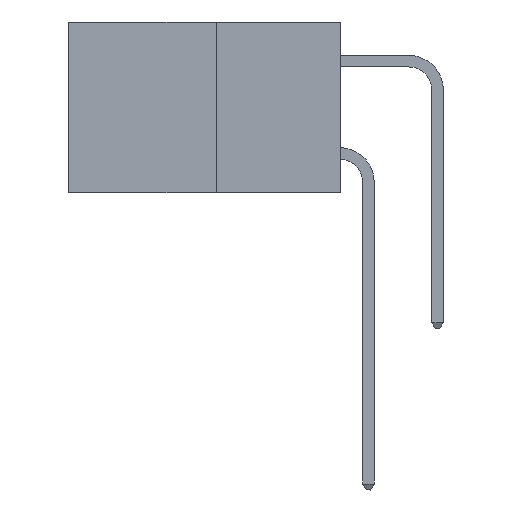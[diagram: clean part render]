
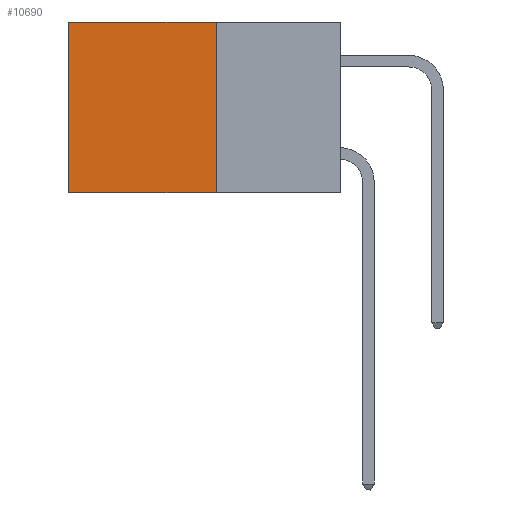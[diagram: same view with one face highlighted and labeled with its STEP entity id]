
A CAD part, left-side view. The second image highlights one B-rep face of the part: STEP entity #10690.
In plain terms, the highlighted planar face has unit normal (-1, 0, 0).
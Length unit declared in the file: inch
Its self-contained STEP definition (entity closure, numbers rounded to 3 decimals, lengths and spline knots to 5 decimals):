
#396 = VECTOR ( 'NONE', #9815, 39.37008 ) ;
#742 = LINE ( 'NONE', #11860, #396 ) ;
#830 = CARTESIAN_POINT ( 'NONE',  ( 0.277, 0.27, 0. ) ) ;
#871 = VECTOR ( 'NONE', #12965, 39.37008 ) ;
#910 = LINE ( 'NONE', #12043, #7142 ) ;
#1106 = CARTESIAN_POINT ( 'NONE',  ( 0.277, 0.59, -0.37 ) ) ;
#1610 = CARTESIAN_POINT ( 'NONE',  ( 0.277, 0.27, -0.37 ) ) ;
#1911 = CARTESIAN_POINT ( 'NONE',  ( 0.277, 0.27, -0.37 ) ) ;
#3246 = DIRECTION ( 'NONE',  ( 1., 0., 0. ) ) ;
#3521 = ORIENTED_EDGE ( 'NONE', *, *, #8546, .T. ) ;
#6115 = VERTEX_POINT ( 'NONE', #1106 ) ;
#6602 = VECTOR ( 'NONE', #10240, 39.37008 ) ;
#6980 = AXIS2_PLACEMENT_3D ( 'NONE', #10043, #3246, #11067 ) ;
#7105 = LINE ( 'NONE', #1911, #871 ) ;
#7142 = VECTOR ( 'NONE', #12002, 39.37008 ) ;
#7728 = EDGE_CURVE ( 'NONE', #10656, #13367, #910, .T. ) ;
#7829 = ORIENTED_EDGE ( 'NONE', *, *, #13526, .F. ) ;
#7856 = PLANE ( 'NONE',  #6980 ) ;
#7890 = CARTESIAN_POINT ( 'NONE',  ( 0.277, 0.59, 0. ) ) ;
#7922 = ORIENTED_EDGE ( 'NONE', *, *, #7728, .F. ) ;
#7990 = CARTESIAN_POINT ( 'NONE',  ( 0.277, 0.59, -0.37 ) ) ;
#8546 = EDGE_CURVE ( 'NONE', #14292, #6115, #9184, .T. ) ;
#9184 = LINE ( 'NONE', #7990, #6602 ) ;
#9752 = ORIENTED_EDGE ( 'NONE', *, *, #11866, .T. ) ;
#9815 = DIRECTION ( 'NONE',  ( 0., 1., 0. ) ) ;
#10043 = CARTESIAN_POINT ( 'NONE',  ( 0.277, 0.27, -0.37 ) ) ;
#10128 = EDGE_LOOP ( 'NONE', ( #3521, #7829, #7922, #9752 ) ) ;
#10240 = DIRECTION ( 'NONE',  ( 0., 0., -1. ) ) ;
#10656 = VERTEX_POINT ( 'NONE', #830 ) ;
#10690 = ADVANCED_FACE ( 'NONE', ( #13609 ), #7856, .F. ) ;
#11067 = DIRECTION ( 'NONE',  ( 0., 0., -1. ) ) ;
#11860 = CARTESIAN_POINT ( 'NONE',  ( 0.277, 0.27, 0. ) ) ;
#11866 = EDGE_CURVE ( 'NONE', #10656, #14292, #742, .T. ) ;
#12002 = DIRECTION ( 'NONE',  ( 0., 0., -1. ) ) ;
#12043 = CARTESIAN_POINT ( 'NONE',  ( 0.277, 0.27, -0.37 ) ) ;
#12965 = DIRECTION ( 'NONE',  ( 0., 1., 0. ) ) ;
#13367 = VERTEX_POINT ( 'NONE', #1610 ) ;
#13526 = EDGE_CURVE ( 'NONE', #13367, #6115, #7105, .T. ) ;
#13609 = FACE_OUTER_BOUND ( 'NONE', #10128, .T. ) ;
#14292 = VERTEX_POINT ( 'NONE', #7890 ) ;
